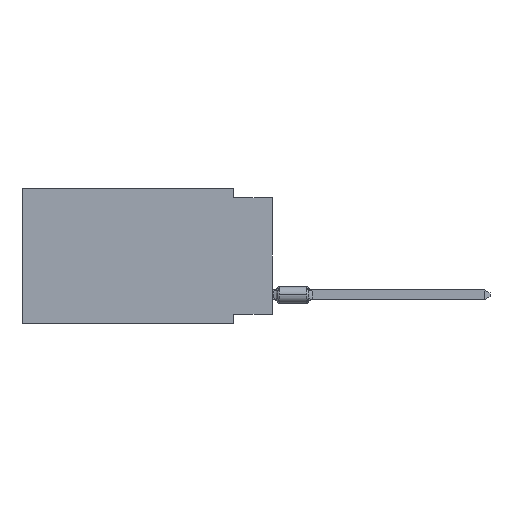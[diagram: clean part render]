
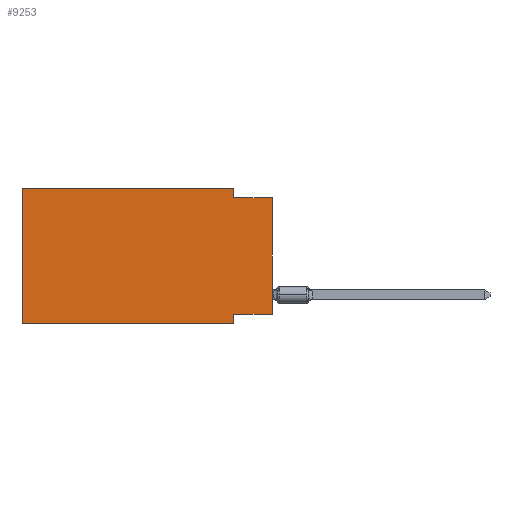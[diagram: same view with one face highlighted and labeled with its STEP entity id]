
A CAD part, left-side view. The second image highlights one B-rep face of the part: STEP entity #9253.
In plain terms, the highlighted planar face has unit normal (-1, 0, 0).
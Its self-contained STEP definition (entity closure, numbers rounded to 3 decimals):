
#141 = VECTOR ( 'NONE', #4885, 1000. ) ;
#150 = ORIENTED_EDGE ( 'NONE', *, *, #2159, .F. ) ;
#278 = VECTOR ( 'NONE', #10987, 1000. ) ;
#301 = CARTESIAN_POINT ( 'NONE',  ( 0., 2.54, -8.89 ) ) ;
#534 = CARTESIAN_POINT ( 'NONE',  ( 0., 0., -0.635 ) ) ;
#654 = VECTOR ( 'NONE', #12161, 1000. ) ;
#730 = CARTESIAN_POINT ( 'NONE',  ( 0., 2.54, -8.89 ) ) ;
#949 = ORIENTED_EDGE ( 'NONE', *, *, #7088, .F. ) ;
#1001 = CARTESIAN_POINT ( 'NONE',  ( 0., 16.383, 0. ) ) ;
#1937 = LINE ( 'NONE', #16351, #278 ) ;
#2159 = EDGE_CURVE ( 'NONE', #4852, #6103, #14898, .T. ) ;
#2473 = EDGE_CURVE ( 'NONE', #14756, #9919, #9443, .T. ) ;
#2737 = CARTESIAN_POINT ( 'NONE',  ( 0., 0., -0.635 ) ) ;
#3563 = VERTEX_POINT ( 'NONE', #15413 ) ;
#3733 = EDGE_CURVE ( 'NONE', #12503, #4852, #13552, .T. ) ;
#3825 = CARTESIAN_POINT ( 'NONE',  ( 0., 16.383, -8.89 ) ) ;
#4646 = CARTESIAN_POINT ( 'NONE',  ( 0., 0., -8.255 ) ) ;
#4686 = DIRECTION ( 'NONE',  ( 0., 0., -1. ) ) ;
#4852 = VERTEX_POINT ( 'NONE', #6113 ) ;
#4885 = DIRECTION ( 'NONE',  ( 0., -1., 0. ) ) ;
#5015 = DIRECTION ( 'NONE',  ( 0., -1., 0. ) ) ;
#5031 = ORIENTED_EDGE ( 'NONE', *, *, #8257, .F. ) ;
#5587 = DIRECTION ( 'NONE',  ( 0., 1., 0. ) ) ;
#5626 = PLANE ( 'NONE',  #9052 ) ;
#5700 = ORIENTED_EDGE ( 'NONE', *, *, #2473, .F. ) ;
#6103 = VERTEX_POINT ( 'NONE', #10781 ) ;
#6113 = CARTESIAN_POINT ( 'NONE',  ( 0., 16.383, 0. ) ) ;
#6782 = ORIENTED_EDGE ( 'NONE', *, *, #14783, .F. ) ;
#6878 = FACE_OUTER_BOUND ( 'NONE', #13693, .T. ) ;
#7008 = DIRECTION ( 'NONE',  ( 0., 0., -1. ) ) ;
#7088 = EDGE_CURVE ( 'NONE', #3563, #8211, #9486, .T. ) ;
#7120 = CARTESIAN_POINT ( 'NONE',  ( 0., 0., 0. ) ) ;
#7464 = LINE ( 'NONE', #7120, #11401 ) ;
#8211 = VERTEX_POINT ( 'NONE', #2737 ) ;
#8257 = EDGE_CURVE ( 'NONE', #12871, #14756, #11693, .T. ) ;
#9052 = AXIS2_PLACEMENT_3D ( 'NONE', #9647, #12320, #4686 ) ;
#9253 = ADVANCED_FACE ( 'NONE', ( #6878 ), #5626, .F. ) ;
#9443 = LINE ( 'NONE', #730, #12998 ) ;
#9486 = LINE ( 'NONE', #534, #654 ) ;
#9647 = CARTESIAN_POINT ( 'NONE',  ( 0., 16.383, 0. ) ) ;
#9919 = VERTEX_POINT ( 'NONE', #301 ) ;
#10068 = VECTOR ( 'NONE', #5015, 1000. ) ;
#10230 = EDGE_CURVE ( 'NONE', #12503, #9919, #12839, .T. ) ;
#10781 = CARTESIAN_POINT ( 'NONE',  ( 0., 2.54, 0. ) ) ;
#10987 = DIRECTION ( 'NONE',  ( 0., 0., -1. ) ) ;
#11401 = VECTOR ( 'NONE', #15071, 1000. ) ;
#11511 = EDGE_CURVE ( 'NONE', #12871, #8211, #7464, .T. ) ;
#11693 = LINE ( 'NONE', #15876, #13043 ) ;
#12161 = DIRECTION ( 'NONE',  ( 0., -1., 0. ) ) ;
#12320 = DIRECTION ( 'NONE',  ( 1., 0., 0. ) ) ;
#12464 = VECTOR ( 'NONE', #15137, 1000. ) ;
#12503 = VERTEX_POINT ( 'NONE', #3825 ) ;
#12839 = LINE ( 'NONE', #13931, #141 ) ;
#12871 = VERTEX_POINT ( 'NONE', #4646 ) ;
#12908 = ORIENTED_EDGE ( 'NONE', *, *, #3733, .F. ) ;
#12998 = VECTOR ( 'NONE', #7008, 1000. ) ;
#13043 = VECTOR ( 'NONE', #5587, 1000. ) ;
#13261 = ORIENTED_EDGE ( 'NONE', *, *, #11511, .T. ) ;
#13457 = ORIENTED_EDGE ( 'NONE', *, *, #10230, .T. ) ;
#13552 = LINE ( 'NONE', #1001, #12464 ) ;
#13693 = EDGE_LOOP ( 'NONE', ( #13261, #949, #6782, #150, #12908, #13457, #5700, #5031 ) ) ;
#13931 = CARTESIAN_POINT ( 'NONE',  ( 0., 16.383, -8.89 ) ) ;
#14756 = VERTEX_POINT ( 'NONE', #15930 ) ;
#14783 = EDGE_CURVE ( 'NONE', #6103, #3563, #1937, .T. ) ;
#14898 = LINE ( 'NONE', #16492, #10068 ) ;
#15071 = DIRECTION ( 'NONE',  ( 0., 0., 1. ) ) ;
#15137 = DIRECTION ( 'NONE',  ( 0., 0., 1. ) ) ;
#15413 = CARTESIAN_POINT ( 'NONE',  ( 0., 2.54, -0.635 ) ) ;
#15876 = CARTESIAN_POINT ( 'NONE',  ( 0., 0., -8.255 ) ) ;
#15930 = CARTESIAN_POINT ( 'NONE',  ( 0., 2.54, -8.255 ) ) ;
#16351 = CARTESIAN_POINT ( 'NONE',  ( 0., 2.54, 0. ) ) ;
#16492 = CARTESIAN_POINT ( 'NONE',  ( 0., 16.383, 0. ) ) ;
